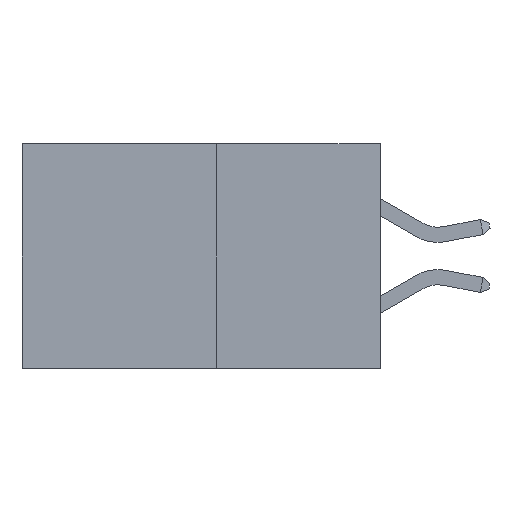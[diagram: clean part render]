
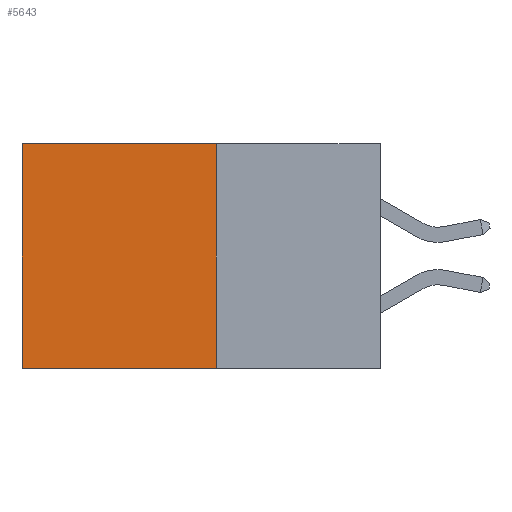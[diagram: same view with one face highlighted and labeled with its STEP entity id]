
A CAD part, left-side view. The second image highlights one B-rep face of the part: STEP entity #5643.
In plain terms, the highlighted planar face has unit normal (-1, 0, 0).
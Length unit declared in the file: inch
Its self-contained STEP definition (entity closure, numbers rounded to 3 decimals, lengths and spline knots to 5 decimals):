
#385 = DIRECTION ( 'NONE',  ( 0., 1., 0. ) ) ;
#1534 = DIRECTION ( 'NONE',  ( 0., 0., -1. ) ) ;
#1694 = ORIENTED_EDGE ( 'NONE', *, *, #11826, .T. ) ;
#1947 = CARTESIAN_POINT ( 'NONE',  ( 0.277, 0.59, 0. ) ) ;
#3085 = VERTEX_POINT ( 'NONE', #6025 ) ;
#3960 = LINE ( 'NONE', #8223, #10739 ) ;
#4920 = ORIENTED_EDGE ( 'NONE', *, *, #10393, .F. ) ;
#5643 = ADVANCED_FACE ( 'NONE', ( #16810 ), #16657, .F. ) ;
#5892 = DIRECTION ( 'NONE',  ( 1., 0., 0. ) ) ;
#6025 = CARTESIAN_POINT ( 'NONE',  ( 0.277, 0.27, 0. ) ) ;
#6181 = CARTESIAN_POINT ( 'NONE',  ( 0.277, 0.59, -0.37 ) ) ;
#6298 = VERTEX_POINT ( 'NONE', #14546 ) ;
#6544 = AXIS2_PLACEMENT_3D ( 'NONE', #12642, #5892, #15385 ) ;
#7294 = VECTOR ( 'NONE', #1534, 39.37008 ) ;
#7713 = LINE ( 'NONE', #15065, #7294 ) ;
#8223 = CARTESIAN_POINT ( 'NONE',  ( 0.277, 0.27, -0.37 ) ) ;
#9623 = VECTOR ( 'NONE', #385, 39.37008 ) ;
#10116 = EDGE_LOOP ( 'NONE', ( #12876, #4920, #15540, #1694 ) ) ;
#10393 = EDGE_CURVE ( 'NONE', #6298, #14407, #3960, .T. ) ;
#10615 = VERTEX_POINT ( 'NONE', #1947 ) ;
#10739 = VECTOR ( 'NONE', #13699, 39.37008 ) ;
#11217 = CARTESIAN_POINT ( 'NONE',  ( 0.277, 0.27, 0. ) ) ;
#11678 = CARTESIAN_POINT ( 'NONE',  ( 0.277, 0.59, -0.37 ) ) ;
#11826 = EDGE_CURVE ( 'NONE', #3085, #10615, #13247, .T. ) ;
#12175 = EDGE_CURVE ( 'NONE', #3085, #6298, #7713, .T. ) ;
#12642 = CARTESIAN_POINT ( 'NONE',  ( 0.277, 0.27, -0.37 ) ) ;
#12876 = ORIENTED_EDGE ( 'NONE', *, *, #16598, .T. ) ;
#12945 = DIRECTION ( 'NONE',  ( 0., 0., -1. ) ) ;
#12965 = LINE ( 'NONE', #6181, #16553 ) ;
#13247 = LINE ( 'NONE', #11217, #9623 ) ;
#13699 = DIRECTION ( 'NONE',  ( 0., 1., 0. ) ) ;
#14407 = VERTEX_POINT ( 'NONE', #11678 ) ;
#14546 = CARTESIAN_POINT ( 'NONE',  ( 0.277, 0.27, -0.37 ) ) ;
#15065 = CARTESIAN_POINT ( 'NONE',  ( 0.277, 0.27, -0.37 ) ) ;
#15385 = DIRECTION ( 'NONE',  ( 0., 0., -1. ) ) ;
#15540 = ORIENTED_EDGE ( 'NONE', *, *, #12175, .F. ) ;
#16553 = VECTOR ( 'NONE', #12945, 39.37008 ) ;
#16598 = EDGE_CURVE ( 'NONE', #10615, #14407, #12965, .T. ) ;
#16657 = PLANE ( 'NONE',  #6544 ) ;
#16810 = FACE_OUTER_BOUND ( 'NONE', #10116, .T. ) ;
